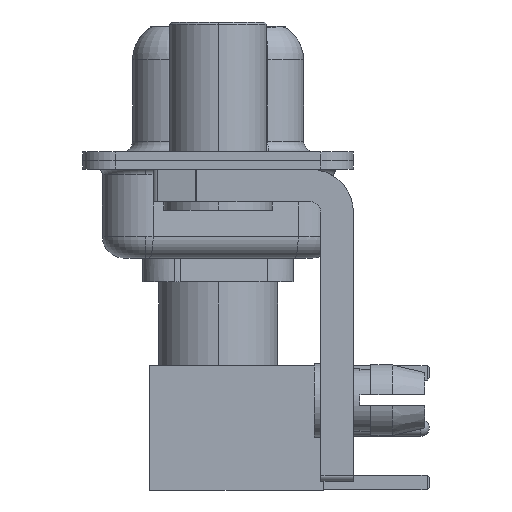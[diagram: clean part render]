
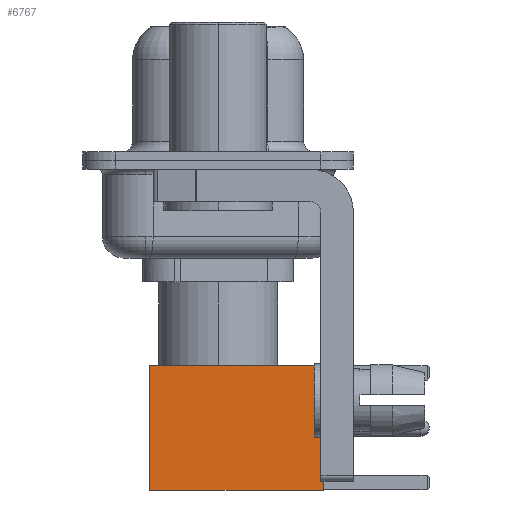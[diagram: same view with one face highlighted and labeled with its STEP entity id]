
A CAD part, left-side view. The second image highlights one B-rep face of the part: STEP entity #6767.
In plain terms, the highlighted face is planar.
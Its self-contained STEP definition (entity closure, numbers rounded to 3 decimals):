
#249 = VERTEX_POINT ( 'NONE', #18400 ) ;
#750 = VERTEX_POINT ( 'NONE', #16185 ) ;
#1120 = ORIENTED_EDGE ( 'NONE', *, *, #18506, .T. ) ;
#1807 = DIRECTION ( 'NONE',  ( 0., 1., 0. ) ) ;
#2415 = VECTOR ( 'NONE', #19758, 1000. ) ;
#3412 = VERTEX_POINT ( 'NONE', #20130 ) ;
#3637 = LINE ( 'NONE', #13962, #19134 ) ;
#3858 = CARTESIAN_POINT ( 'NONE',  ( 0., 2.875, 8. ) ) ;
#4065 = DIRECTION ( 'NONE',  ( -1., 0., 0. ) ) ;
#4761 = CARTESIAN_POINT ( 'NONE',  ( 2.875, 2.875, 0. ) ) ;
#5813 = EDGE_CURVE ( 'NONE', #3412, #249, #13112, .T. ) ;
#5827 = LINE ( 'NONE', #3858, #14425 ) ;
#6237 = ORIENTED_EDGE ( 'NONE', *, *, #5813, .T. ) ;
#6767 = ADVANCED_FACE ( 'NONE', ( #20220 ), #18456, .T. ) ;
#7751 = EDGE_CURVE ( 'NONE', #9075, #750, #3637, .T. ) ;
#9075 = VERTEX_POINT ( 'NONE', #10723 ) ;
#10593 = EDGE_CURVE ( 'NONE', #3412, #9075, #5827, .T. ) ;
#10723 = CARTESIAN_POINT ( 'NONE',  ( -2.875, 2.875, 8. ) ) ;
#11988 = ORIENTED_EDGE ( 'NONE', *, *, #7751, .F. ) ;
#12088 = DIRECTION ( 'NONE',  ( 0., 0., -1. ) ) ;
#12726 = AXIS2_PLACEMENT_3D ( 'NONE', #13358, #1807, #16885 ) ;
#13112 = LINE ( 'NONE', #4761, #2415 ) ;
#13358 = CARTESIAN_POINT ( 'NONE',  ( 2.875, 2.875, 0. ) ) ;
#13579 = EDGE_LOOP ( 'NONE', ( #6237, #1120, #11988, #15219 ) ) ;
#13962 = CARTESIAN_POINT ( 'NONE',  ( -2.875, 2.875, 0. ) ) ;
#14107 = CARTESIAN_POINT ( 'NONE',  ( 0., 2.875, 0. ) ) ;
#14425 = VECTOR ( 'NONE', #4065, 1000. ) ;
#14578 = VECTOR ( 'NONE', #15987, 1000. ) ;
#15219 = ORIENTED_EDGE ( 'NONE', *, *, #10593, .F. ) ;
#15987 = DIRECTION ( 'NONE',  ( -1., 0., 0. ) ) ;
#16185 = CARTESIAN_POINT ( 'NONE',  ( -2.875, 2.875, 0. ) ) ;
#16885 = DIRECTION ( 'NONE',  ( 0., 0., 1. ) ) ;
#17643 = LINE ( 'NONE', #14107, #14578 ) ;
#18400 = CARTESIAN_POINT ( 'NONE',  ( 2.875, 2.875, 0. ) ) ;
#18456 = PLANE ( 'NONE',  #12726 ) ;
#18506 = EDGE_CURVE ( 'NONE', #249, #750, #17643, .T. ) ;
#19134 = VECTOR ( 'NONE', #12088, 1000. ) ;
#19758 = DIRECTION ( 'NONE',  ( 0., 0., -1. ) ) ;
#20130 = CARTESIAN_POINT ( 'NONE',  ( 2.875, 2.875, 8. ) ) ;
#20220 = FACE_OUTER_BOUND ( 'NONE', #13579, .T. ) ;
